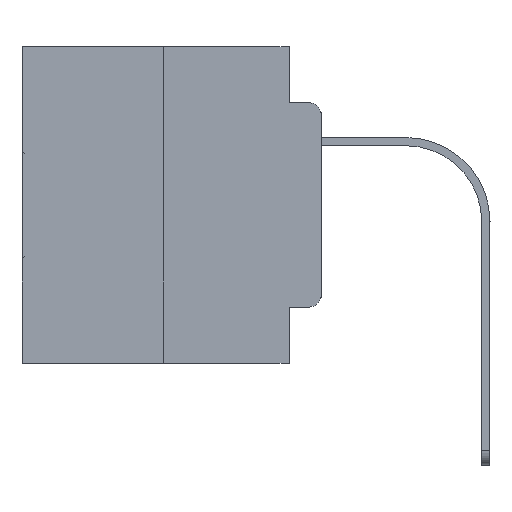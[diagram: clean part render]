
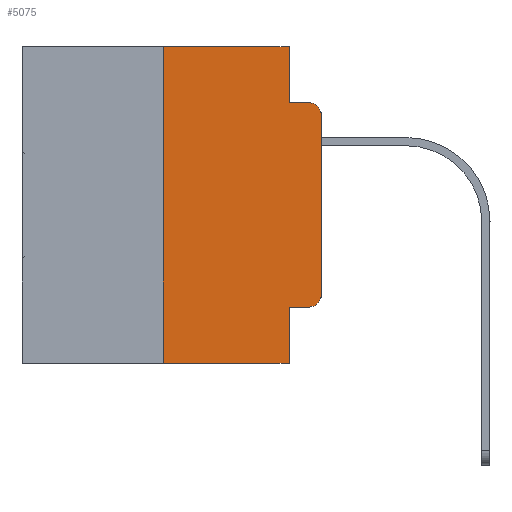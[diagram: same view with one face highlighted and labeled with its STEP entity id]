
A CAD part, left-side view. The second image highlights one B-rep face of the part: STEP entity #5075.
In plain terms, the highlighted planar face has unit normal (-1, 0, 0).
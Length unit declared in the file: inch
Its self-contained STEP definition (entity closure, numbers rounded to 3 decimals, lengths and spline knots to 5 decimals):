
#310 = CARTESIAN_POINT ( 'NONE',  ( 0., 0.25, 0. ) ) ;
#1051 = CARTESIAN_POINT ( 'NONE',  ( 0., 0.473, 0. ) ) ;
#2182 = CARTESIAN_POINT ( 'NONE',  ( 0., 0.02, -0.0885 ) ) ;
#2482 = CARTESIAN_POINT ( 'NONE',  ( 0., 0.051, -0.0885 ) ) ;
#3563 = ORIENTED_EDGE ( 'NONE', *, *, #7248, .T. ) ;
#4004 = DIRECTION ( 'NONE',  ( 0., 0., 1. ) ) ;
#4725 = VERTEX_POINT ( 'NONE', #5787 ) ;
#4797 = VECTOR ( 'NONE', #7597, 39.37008 ) ;
#5075 = ADVANCED_FACE ( 'NONE', ( #19153 ), #28270, .F. ) ;
#5364 = AXIS2_PLACEMENT_3D ( 'NONE', #24620, #18196, #27316 ) ;
#5398 = ORIENTED_EDGE ( 'NONE', *, *, #10416, .T. ) ;
#5787 = CARTESIAN_POINT ( 'NONE',  ( 0., 0.051, -0.5 ) ) ;
#6157 = VECTOR ( 'NONE', #4004, 39.37008 ) ;
#6525 = LINE ( 'NONE', #15073, #6157 ) ;
#6727 = VECTOR ( 'NONE', #23733, 39.37008 ) ;
#7248 = EDGE_CURVE ( 'NONE', #25662, #24336, #6525, .T. ) ;
#7271 = VERTEX_POINT ( 'NONE', #17888 ) ;
#7450 = DIRECTION ( 'NONE',  ( 0., 0., 1. ) ) ;
#7529 = EDGE_CURVE ( 'NONE', #7271, #24489, #16132, .T. ) ;
#7597 = DIRECTION ( 'NONE',  ( 0., 0., -1. ) ) ;
#7824 = CARTESIAN_POINT ( 'NONE',  ( 0., 0.473, 0. ) ) ;
#7983 = VECTOR ( 'NONE', #7450, 39.37008 ) ;
#8314 = CARTESIAN_POINT ( 'NONE',  ( 0., 0.25, 0. ) ) ;
#8523 = CARTESIAN_POINT ( 'NONE',  ( 0., 0.473, -0.5 ) ) ;
#8674 = ORIENTED_EDGE ( 'NONE', *, *, #23686, .T. ) ;
#8689 = AXIS2_PLACEMENT_3D ( 'NONE', #15908, #15473, #27099 ) ;
#8724 = EDGE_CURVE ( 'NONE', #20267, #4725, #16137, .T. ) ;
#8911 = EDGE_CURVE ( 'NONE', #20267, #24465, #28657, .T. ) ;
#9185 = VECTOR ( 'NONE', #17468, 39.37008 ) ;
#10104 = CARTESIAN_POINT ( 'NONE',  ( 0., 0., -0.3915 ) ) ;
#10416 = EDGE_CURVE ( 'NONE', #24336, #24222, #19669, .T. ) ;
#10653 = DIRECTION ( 'NONE',  ( 0., 0., -1. ) ) ;
#11749 = LINE ( 'NONE', #20835, #26631 ) ;
#11882 = CARTESIAN_POINT ( 'NONE',  ( 0., 0., -0.1085 ) ) ;
#12244 = ORIENTED_EDGE ( 'NONE', *, *, #24656, .T. ) ;
#12321 = ORIENTED_EDGE ( 'NONE', *, *, #8911, .T. ) ;
#12780 = CARTESIAN_POINT ( 'NONE',  ( 0., 0.02, -0.4115 ) ) ;
#12836 = VECTOR ( 'NONE', #13717, 39.37008 ) ;
#13484 = EDGE_CURVE ( 'NONE', #24489, #28018, #28821, .T. ) ;
#13717 = DIRECTION ( 'NONE',  ( 0., -1., 0. ) ) ;
#14346 = CARTESIAN_POINT ( 'NONE',  ( 0., 0.051, 0. ) ) ;
#15055 = ORIENTED_EDGE ( 'NONE', *, *, #21545, .F. ) ;
#15073 = CARTESIAN_POINT ( 'NONE',  ( 0., 0., 0. ) ) ;
#15473 = DIRECTION ( 'NONE',  ( -1., 0., 0. ) ) ;
#15659 = CARTESIAN_POINT ( 'NONE',  ( 0., 0.051, -0.0885 ) ) ;
#15908 = CARTESIAN_POINT ( 'NONE',  ( 0., 0.02, -0.3915 ) ) ;
#16132 = LINE ( 'NONE', #310, #7983 ) ;
#16137 = LINE ( 'NONE', #14346, #4797 ) ;
#16742 = VECTOR ( 'NONE', #26889, 39.37008 ) ;
#16799 = AXIS2_PLACEMENT_3D ( 'NONE', #7824, #16924, #10653 ) ;
#16924 = DIRECTION ( 'NONE',  ( 1., 0., 0. ) ) ;
#17468 = DIRECTION ( 'NONE',  ( 0., -1., 0. ) ) ;
#17869 = CARTESIAN_POINT ( 'NONE',  ( 0., 0.051, 0. ) ) ;
#17888 = CARTESIAN_POINT ( 'NONE',  ( 0., 0.25, -0.5 ) ) ;
#18196 = DIRECTION ( 'NONE',  ( -1., 0., 0. ) ) ;
#18217 = CIRCLE ( 'NONE', #8689, 0.02 ) ;
#19153 = FACE_OUTER_BOUND ( 'NONE', #26467, .T. ) ;
#19669 = CIRCLE ( 'NONE', #5364, 0.02 ) ;
#20247 = EDGE_CURVE ( 'NONE', #22681, #24222, #25040, .T. ) ;
#20267 = VERTEX_POINT ( 'NONE', #22495 ) ;
#20835 = CARTESIAN_POINT ( 'NONE',  ( 0., 0.051, 0. ) ) ;
#21451 = ORIENTED_EDGE ( 'NONE', *, *, #13484, .F. ) ;
#21545 = EDGE_CURVE ( 'NONE', #28018, #22681, #11749, .T. ) ;
#21599 = ORIENTED_EDGE ( 'NONE', *, *, #8724, .F. ) ;
#21941 = LINE ( 'NONE', #8523, #16742 ) ;
#22318 = ORIENTED_EDGE ( 'NONE', *, *, #7529, .F. ) ;
#22495 = CARTESIAN_POINT ( 'NONE',  ( 0., 0.051, -0.4115 ) ) ;
#22681 = VERTEX_POINT ( 'NONE', #15659 ) ;
#23686 = EDGE_CURVE ( 'NONE', #7271, #4725, #21941, .T. ) ;
#23733 = DIRECTION ( 'NONE',  ( 0., -1., 0. ) ) ;
#24222 = VERTEX_POINT ( 'NONE', #2182 ) ;
#24336 = VERTEX_POINT ( 'NONE', #11882 ) ;
#24465 = VERTEX_POINT ( 'NONE', #12780 ) ;
#24489 = VERTEX_POINT ( 'NONE', #8314 ) ;
#24620 = CARTESIAN_POINT ( 'NONE',  ( 0., 0.02, -0.1085 ) ) ;
#24656 = EDGE_CURVE ( 'NONE', #24465, #25662, #18217, .T. ) ;
#25040 = LINE ( 'NONE', #2482, #12836 ) ;
#25662 = VERTEX_POINT ( 'NONE', #10104 ) ;
#26467 = EDGE_LOOP ( 'NONE', ( #3563, #5398, #28594, #15055, #21451, #22318, #8674, #21599, #12321, #12244 ) ) ;
#26631 = VECTOR ( 'NONE', #27725, 39.37008 ) ;
#26889 = DIRECTION ( 'NONE',  ( 0., -1., 0. ) ) ;
#27099 = DIRECTION ( 'NONE',  ( 0., 0., -1. ) ) ;
#27316 = DIRECTION ( 'NONE',  ( 0., 0., -1. ) ) ;
#27725 = DIRECTION ( 'NONE',  ( 0., 0., -1. ) ) ;
#28018 = VERTEX_POINT ( 'NONE', #17869 ) ;
#28270 = PLANE ( 'NONE',  #16799 ) ;
#28366 = CARTESIAN_POINT ( 'NONE',  ( 0., 0.051, -0.4115 ) ) ;
#28594 = ORIENTED_EDGE ( 'NONE', *, *, #20247, .F. ) ;
#28657 = LINE ( 'NONE', #28366, #6727 ) ;
#28821 = LINE ( 'NONE', #1051, #9185 ) ;
